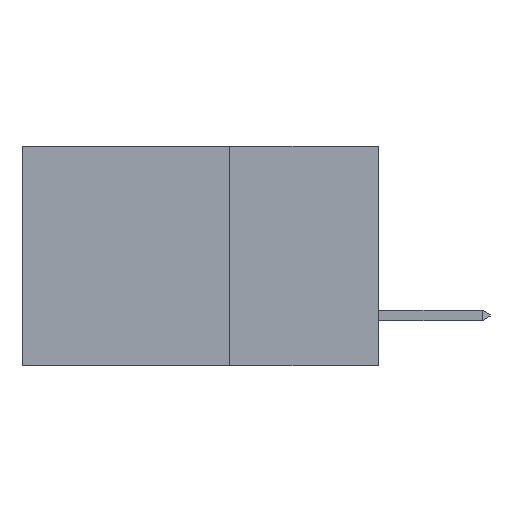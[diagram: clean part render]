
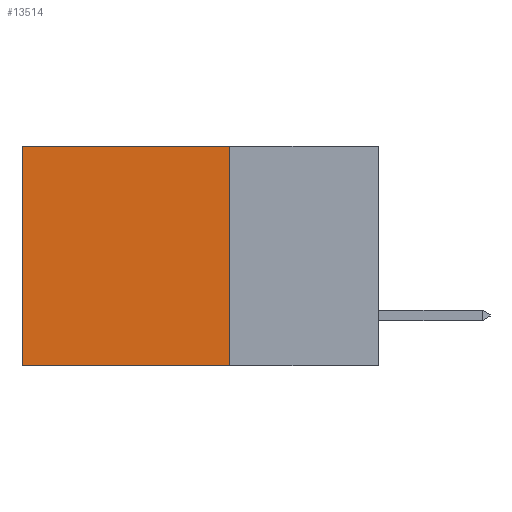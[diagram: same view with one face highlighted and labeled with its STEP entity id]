
A CAD part, left-side view. The second image highlights one B-rep face of the part: STEP entity #13514.
In plain terms, the highlighted planar face has unit normal (-1, 0, 0).
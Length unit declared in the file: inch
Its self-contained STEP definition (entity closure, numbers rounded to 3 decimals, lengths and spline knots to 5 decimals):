
#83 = DIRECTION ( 'NONE',  ( 0., 1., 0. ) ) ;
#156 = AXIS2_PLACEMENT_3D ( 'NONE', #22445, #19238, #8171 ) ;
#368 = ORIENTED_EDGE ( 'NONE', *, *, #10169, .T. ) ;
#734 = LINE ( 'NONE', #5033, #10190 ) ;
#1252 = EDGE_CURVE ( 'NONE', #14449, #7186, #734, .T. ) ;
#2107 = EDGE_CURVE ( 'NONE', #22683, #12115, #15424, .T. ) ;
#2571 = CARTESIAN_POINT ( 'NONE',  ( 0.298, 0.6, 0. ) ) ;
#2719 = EDGE_LOOP ( 'NONE', ( #368, #4032, #15367, #22481 ) ) ;
#3596 = VECTOR ( 'NONE', #20179, 39.37008 ) ;
#4032 = ORIENTED_EDGE ( 'NONE', *, *, #2107, .F. ) ;
#5033 = CARTESIAN_POINT ( 'NONE',  ( 0.298, 0.25, 0. ) ) ;
#7186 = VERTEX_POINT ( 'NONE', #11282 ) ;
#7253 = CARTESIAN_POINT ( 'NONE',  ( 0.298, 0.25, 0. ) ) ;
#7261 = CARTESIAN_POINT ( 'NONE',  ( 0.298, 0.6, -0.37 ) ) ;
#8171 = DIRECTION ( 'NONE',  ( 0., 0., -1. ) ) ;
#8513 = FACE_OUTER_BOUND ( 'NONE', #2719, .T. ) ;
#10169 = EDGE_CURVE ( 'NONE', #7186, #12115, #16280, .T. ) ;
#10190 = VECTOR ( 'NONE', #13690, 39.37008 ) ;
#11282 = CARTESIAN_POINT ( 'NONE',  ( 0.298, 0.6, 0. ) ) ;
#12115 = VERTEX_POINT ( 'NONE', #7261 ) ;
#13514 = ADVANCED_FACE ( 'NONE', ( #8513 ), #18878, .F. ) ;
#13690 = DIRECTION ( 'NONE',  ( 0., 1., 0. ) ) ;
#14449 = VERTEX_POINT ( 'NONE', #23872 ) ;
#15367 = ORIENTED_EDGE ( 'NONE', *, *, #19527, .F. ) ;
#15424 = LINE ( 'NONE', #15455, #19685 ) ;
#15455 = CARTESIAN_POINT ( 'NONE',  ( 0.298, 0.25, -0.37 ) ) ;
#15645 = DIRECTION ( 'NONE',  ( 0., 0., -1. ) ) ;
#16280 = LINE ( 'NONE', #2571, #16870 ) ;
#16870 = VECTOR ( 'NONE', #15645, 39.37008 ) ;
#17679 = CARTESIAN_POINT ( 'NONE',  ( 0.298, 0.25, -0.37 ) ) ;
#18500 = LINE ( 'NONE', #7253, #3596 ) ;
#18878 = PLANE ( 'NONE',  #156 ) ;
#19238 = DIRECTION ( 'NONE',  ( 1., 0., 0. ) ) ;
#19527 = EDGE_CURVE ( 'NONE', #14449, #22683, #18500, .T. ) ;
#19685 = VECTOR ( 'NONE', #83, 39.37008 ) ;
#20179 = DIRECTION ( 'NONE',  ( 0., 0., -1. ) ) ;
#22445 = CARTESIAN_POINT ( 'NONE',  ( 0.298, 0.25, 0. ) ) ;
#22481 = ORIENTED_EDGE ( 'NONE', *, *, #1252, .T. ) ;
#22683 = VERTEX_POINT ( 'NONE', #17679 ) ;
#23872 = CARTESIAN_POINT ( 'NONE',  ( 0.298, 0.25, 0. ) ) ;
